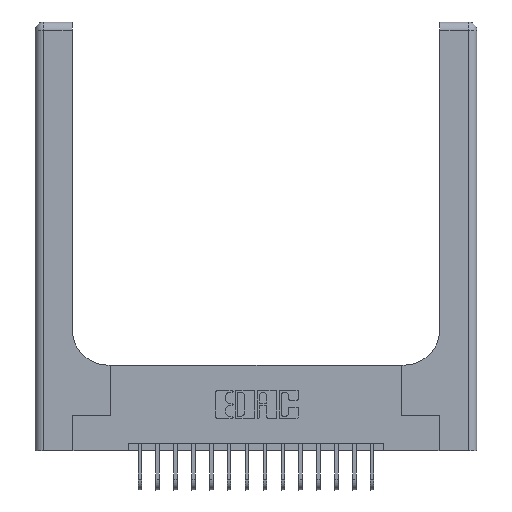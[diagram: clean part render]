
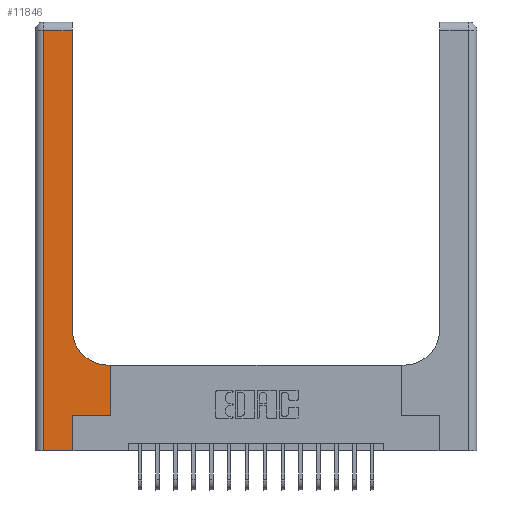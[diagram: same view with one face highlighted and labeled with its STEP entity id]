
A CAD part, top view. The second image highlights one B-rep face of the part: STEP entity #11846.
In plain terms, the highlighted planar face has unit normal (0, 0, 1).
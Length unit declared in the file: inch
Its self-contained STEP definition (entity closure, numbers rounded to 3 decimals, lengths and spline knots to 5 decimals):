
#110 = VECTOR ( 'NONE', #12128, 39.37008 ) ;
#128 = VERTEX_POINT ( 'NONE', #15751 ) ;
#488 = CARTESIAN_POINT ( 'NONE',  ( 0.528, 0.6, 0.37 ) ) ;
#547 = ORIENTED_EDGE ( 'NONE', *, *, #7130, .T. ) ;
#571 = DIRECTION ( 'NONE',  ( 0., 0., -1. ) ) ;
#573 = DIRECTION ( 'NONE',  ( 0., 1., 0. ) ) ;
#625 = CARTESIAN_POINT ( 'NONE',  ( 0.26, 0.6, 0.37 ) ) ;
#663 = DIRECTION ( 'NONE',  ( 1., 0., 0. ) ) ;
#910 = CARTESIAN_POINT ( 'NONE',  ( 0.265, 0.25, 0.37 ) ) ;
#931 = CARTESIAN_POINT ( 'NONE',  ( 0.51, 0.85, 0.37 ) ) ;
#950 = AXIS2_PLACEMENT_3D ( 'NONE', #7732, #571, #3514 ) ;
#962 = CIRCLE ( 'NONE', #5675, 0.25 ) ;
#1008 = CARTESIAN_POINT ( 'NONE',  ( 0.26, 3., 0.37 ) ) ;
#1088 = LINE ( 'NONE', #12662, #9520 ) ;
#1640 = EDGE_CURVE ( 'NONE', #18073, #6395, #962, .T. ) ;
#2004 = CARTESIAN_POINT ( 'NONE',  ( 0., 2.94, 0.37 ) ) ;
#2026 = LINE ( 'NONE', #17455, #110 ) ;
#2488 = LINE ( 'NONE', #1008, #7362 ) ;
#2860 = CARTESIAN_POINT ( 'NONE',  ( 0.265, 0.25, 0.37 ) ) ;
#3057 = PLANE ( 'NONE',  #950 ) ;
#3121 = VERTEX_POINT ( 'NONE', #488 ) ;
#3514 = DIRECTION ( 'NONE',  ( -1., 0., 0. ) ) ;
#3520 = VECTOR ( 'NONE', #10641, 39.37008 ) ;
#3967 = VECTOR ( 'NONE', #573, 39.37008 ) ;
#4520 = EDGE_CURVE ( 'NONE', #15072, #4805, #14164, .T. ) ;
#4805 = VERTEX_POINT ( 'NONE', #17371 ) ;
#4872 = EDGE_CURVE ( 'NONE', #6395, #8297, #2488, .T. ) ;
#5235 = ORIENTED_EDGE ( 'NONE', *, *, #1640, .T. ) ;
#5675 = AXIS2_PLACEMENT_3D ( 'NONE', #931, #11957, #663 ) ;
#6174 = CARTESIAN_POINT ( 'NONE',  ( 0.265, 0., 0.37 ) ) ;
#6395 = VERTEX_POINT ( 'NONE', #13989 ) ;
#7130 = EDGE_CURVE ( 'NONE', #128, #10675, #8055, .T. ) ;
#7322 = DIRECTION ( 'NONE',  ( -1., 0., 0. ) ) ;
#7362 = VECTOR ( 'NONE', #7720, 39.37008 ) ;
#7720 = DIRECTION ( 'NONE',  ( 0., 1., 0. ) ) ;
#7732 = CARTESIAN_POINT ( 'NONE',  ( 0., 3., 0.37 ) ) ;
#8055 = LINE ( 'NONE', #13576, #3520 ) ;
#8073 = VECTOR ( 'NONE', #7322, 39.37008 ) ;
#8225 = EDGE_LOOP ( 'NONE', ( #12587, #16787, #8498, #547, #16089, #13495, #16675, #12450, #5235 ) ) ;
#8297 = VERTEX_POINT ( 'NONE', #12030 ) ;
#8471 = DIRECTION ( 'NONE',  ( 1., 0., 0. ) ) ;
#8498 = ORIENTED_EDGE ( 'NONE', *, *, #14039, .T. ) ;
#9090 = LINE ( 'NONE', #625, #11271 ) ;
#9222 = LINE ( 'NONE', #6174, #3967 ) ;
#9520 = VECTOR ( 'NONE', #15506, 39.37008 ) ;
#10641 = DIRECTION ( 'NONE',  ( 1., 0., 0. ) ) ;
#10664 = CARTESIAN_POINT ( 'NONE',  ( 0.265, 0., 0.37 ) ) ;
#10675 = VERTEX_POINT ( 'NONE', #10664 ) ;
#11271 = VECTOR ( 'NONE', #17435, 39.37008 ) ;
#11846 = ADVANCED_FACE ( 'NONE', ( #17291 ), #3057, .F. ) ;
#11957 = DIRECTION ( 'NONE',  ( 0., 0., -1. ) ) ;
#12030 = CARTESIAN_POINT ( 'NONE',  ( 0.26, 2.94, 0.37 ) ) ;
#12128 = DIRECTION ( 'NONE',  ( 0., 1., 0. ) ) ;
#12450 = ORIENTED_EDGE ( 'NONE', *, *, #13790, .T. ) ;
#12587 = ORIENTED_EDGE ( 'NONE', *, *, #4872, .T. ) ;
#12662 = CARTESIAN_POINT ( 'NONE',  ( 0.06, 3., 0.37 ) ) ;
#13181 = CARTESIAN_POINT ( 'NONE',  ( 0.51, 0.6, 0.37 ) ) ;
#13289 = VECTOR ( 'NONE', #8471, 39.37008 ) ;
#13406 = EDGE_CURVE ( 'NONE', #4805, #3121, #2026, .T. ) ;
#13495 = ORIENTED_EDGE ( 'NONE', *, *, #4520, .T. ) ;
#13521 = VERTEX_POINT ( 'NONE', #18087 ) ;
#13576 = CARTESIAN_POINT ( 'NONE',  ( 0., 0., 0.37 ) ) ;
#13790 = EDGE_CURVE ( 'NONE', #3121, #18073, #9090, .T. ) ;
#13989 = CARTESIAN_POINT ( 'NONE',  ( 0.26, 0.85, 0.37 ) ) ;
#14039 = EDGE_CURVE ( 'NONE', #13521, #128, #1088, .T. ) ;
#14164 = LINE ( 'NONE', #2860, #13289 ) ;
#14410 = LINE ( 'NONE', #2004, #8073 ) ;
#15072 = VERTEX_POINT ( 'NONE', #910 ) ;
#15506 = DIRECTION ( 'NONE',  ( 0., -1., 0. ) ) ;
#15751 = CARTESIAN_POINT ( 'NONE',  ( 0.06, 0., 0.37 ) ) ;
#16089 = ORIENTED_EDGE ( 'NONE', *, *, #16418, .T. ) ;
#16418 = EDGE_CURVE ( 'NONE', #10675, #15072, #9222, .T. ) ;
#16628 = EDGE_CURVE ( 'NONE', #8297, #13521, #14410, .T. ) ;
#16675 = ORIENTED_EDGE ( 'NONE', *, *, #13406, .T. ) ;
#16787 = ORIENTED_EDGE ( 'NONE', *, *, #16628, .T. ) ;
#17291 = FACE_OUTER_BOUND ( 'NONE', #8225, .T. ) ;
#17371 = CARTESIAN_POINT ( 'NONE',  ( 0.528, 0.25, 0.37 ) ) ;
#17435 = DIRECTION ( 'NONE',  ( -1., 0., 0. ) ) ;
#17455 = CARTESIAN_POINT ( 'NONE',  ( 0.528, 0.25, 0.37 ) ) ;
#18073 = VERTEX_POINT ( 'NONE', #13181 ) ;
#18087 = CARTESIAN_POINT ( 'NONE',  ( 0.06, 2.94, 0.37 ) ) ;
